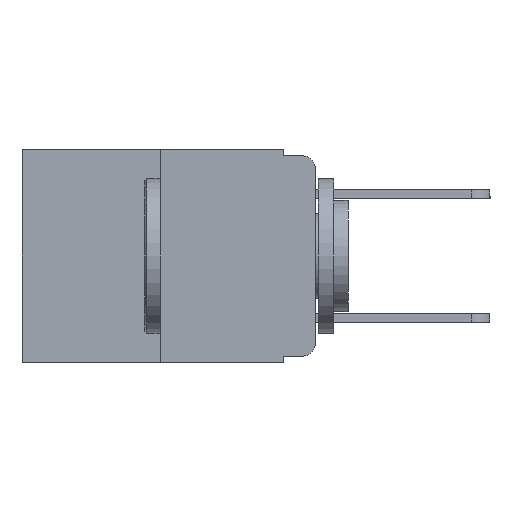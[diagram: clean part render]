
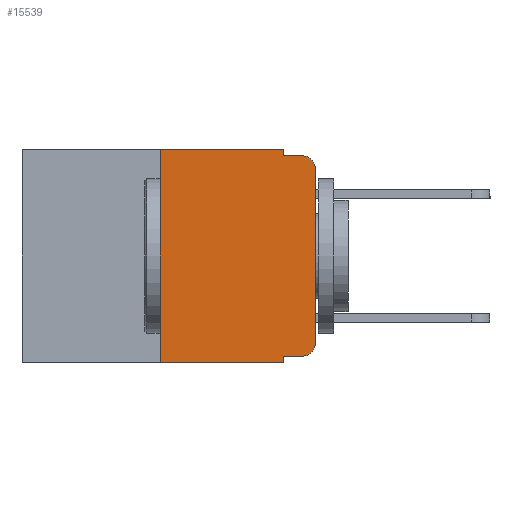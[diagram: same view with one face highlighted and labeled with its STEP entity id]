
A CAD part, left-side view. The second image highlights one B-rep face of the part: STEP entity #15539.
In plain terms, the highlighted planar face has unit normal (-1, 0, 0).
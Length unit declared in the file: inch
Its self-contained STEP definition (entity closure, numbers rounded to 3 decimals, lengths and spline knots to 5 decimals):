
#619 = CARTESIAN_POINT ( 'NONE',  ( 0., 0.02, -0.01 ) ) ;
#672 = VERTEX_POINT ( 'NONE', #3998 ) ;
#719 = VERTEX_POINT ( 'NONE', #619 ) ;
#890 = ORIENTED_EDGE ( 'NONE', *, *, #9875, .T. ) ;
#940 = CARTESIAN_POINT ( 'NONE',  ( 0., 0.051, -0.01 ) ) ;
#1463 = DIRECTION ( 'NONE',  ( -1., 0., 0. ) ) ;
#1755 = DIRECTION ( 'NONE',  ( 0., 0., -1. ) ) ;
#1847 = DIRECTION ( 'NONE',  ( -1., 0., 0. ) ) ;
#2084 = CARTESIAN_POINT ( 'NONE',  ( 0., 0.02, -0.03 ) ) ;
#2374 = LINE ( 'NONE', #5950, #15379 ) ;
#2557 = LINE ( 'NONE', #4442, #19301 ) ;
#2604 = CARTESIAN_POINT ( 'NONE',  ( 0., 0.25, -0.343 ) ) ;
#3172 = AXIS2_PLACEMENT_3D ( 'NONE', #11943, #1463, #13511 ) ;
#3240 = EDGE_CURVE ( 'NONE', #21312, #719, #14729, .T. ) ;
#3321 = PLANE ( 'NONE',  #15184 ) ;
#3429 = VECTOR ( 'NONE', #4644, 39.37008 ) ;
#3998 = CARTESIAN_POINT ( 'NONE',  ( 0., 0.02, -0.333 ) ) ;
#4213 = CARTESIAN_POINT ( 'NONE',  ( 0., 0.25, 0. ) ) ;
#4442 = CARTESIAN_POINT ( 'NONE',  ( 0., 0.051, 0. ) ) ;
#4644 = DIRECTION ( 'NONE',  ( 0., 0., -1. ) ) ;
#4833 = VERTEX_POINT ( 'NONE', #12881 ) ;
#5099 = DIRECTION ( 'NONE',  ( 1., 0., 0. ) ) ;
#5165 = VERTEX_POINT ( 'NONE', #5375 ) ;
#5375 = CARTESIAN_POINT ( 'NONE',  ( 0., 0.051, 0. ) ) ;
#5431 = ORIENTED_EDGE ( 'NONE', *, *, #12209, .T. ) ;
#5826 = ORIENTED_EDGE ( 'NONE', *, *, #19727, .T. ) ;
#5950 = CARTESIAN_POINT ( 'NONE',  ( 0., 0.25, 0. ) ) ;
#5953 = CARTESIAN_POINT ( 'NONE',  ( 0., 0.473, -0.343 ) ) ;
#5994 = CARTESIAN_POINT ( 'NONE',  ( 0., 0.051, -0.333 ) ) ;
#6104 = AXIS2_PLACEMENT_3D ( 'NONE', #2084, #1847, #1755 ) ;
#6261 = ORIENTED_EDGE ( 'NONE', *, *, #11265, .F. ) ;
#6351 = ORIENTED_EDGE ( 'NONE', *, *, #13387, .F. ) ;
#6363 = VERTEX_POINT ( 'NONE', #4213 ) ;
#6409 = ORIENTED_EDGE ( 'NONE', *, *, #3240, .T. ) ;
#6993 = CARTESIAN_POINT ( 'NONE',  ( 0., 0.051, -0.343 ) ) ;
#7061 = FACE_OUTER_BOUND ( 'NONE', #12437, .T. ) ;
#7512 = LINE ( 'NONE', #14798, #3429 ) ;
#7659 = CARTESIAN_POINT ( 'NONE',  ( 0., 0.473, 0. ) ) ;
#7741 = DIRECTION ( 'NONE',  ( 0., 0., 1. ) ) ;
#9471 = DIRECTION ( 'NONE',  ( 0., -1., 0. ) ) ;
#9743 = EDGE_CURVE ( 'NONE', #4833, #18101, #7512, .T. ) ;
#9875 = EDGE_CURVE ( 'NONE', #18501, #21312, #12802, .T. ) ;
#10159 = CARTESIAN_POINT ( 'NONE',  ( 0., 0., -0.313 ) ) ;
#10371 = DIRECTION ( 'NONE',  ( 0., 0., 1. ) ) ;
#10495 = CIRCLE ( 'NONE', #3172, 0.02 ) ;
#10674 = CARTESIAN_POINT ( 'NONE',  ( 0., 0.051, -0.01 ) ) ;
#11265 = EDGE_CURVE ( 'NONE', #5165, #17595, #2557, .T. ) ;
#11751 = LINE ( 'NONE', #940, #19759 ) ;
#11943 = CARTESIAN_POINT ( 'NONE',  ( 0., 0.02, -0.313 ) ) ;
#12209 = EDGE_CURVE ( 'NONE', #672, #18501, #10495, .T. ) ;
#12437 = EDGE_LOOP ( 'NONE', ( #890, #6409, #6351, #6261, #15819, #14343, #15837, #19990, #5826, #5431 ) ) ;
#12802 = LINE ( 'NONE', #21514, #17656 ) ;
#12881 = CARTESIAN_POINT ( 'NONE',  ( 0., 0.051, -0.333 ) ) ;
#13387 = EDGE_CURVE ( 'NONE', #17595, #719, #11751, .T. ) ;
#13511 = DIRECTION ( 'NONE',  ( 0., 0., -1. ) ) ;
#13616 = CARTESIAN_POINT ( 'NONE',  ( 0., 0.473, 0. ) ) ;
#14073 = CARTESIAN_POINT ( 'NONE',  ( 0., 0., -0.03 ) ) ;
#14343 = ORIENTED_EDGE ( 'NONE', *, *, #17214, .F. ) ;
#14729 = CIRCLE ( 'NONE', #6104, 0.02 ) ;
#14737 = DIRECTION ( 'NONE',  ( 0., -1., 0. ) ) ;
#14798 = CARTESIAN_POINT ( 'NONE',  ( 0., 0.051, 0. ) ) ;
#15184 = AXIS2_PLACEMENT_3D ( 'NONE', #13616, #5099, #16923 ) ;
#15379 = VECTOR ( 'NONE', #7741, 39.37008 ) ;
#15539 = ADVANCED_FACE ( 'NONE', ( #7061 ), #3321, .F. ) ;
#15819 = ORIENTED_EDGE ( 'NONE', *, *, #17189, .F. ) ;
#15837 = ORIENTED_EDGE ( 'NONE', *, *, #18880, .T. ) ;
#16193 = VECTOR ( 'NONE', #20798, 39.37008 ) ;
#16714 = LINE ( 'NONE', #5953, #16193 ) ;
#16923 = DIRECTION ( 'NONE',  ( 0., 0., -1. ) ) ;
#16930 = LINE ( 'NONE', #7659, #20121 ) ;
#17189 = EDGE_CURVE ( 'NONE', #6363, #5165, #16930, .T. ) ;
#17214 = EDGE_CURVE ( 'NONE', #18329, #6363, #2374, .T. ) ;
#17595 = VERTEX_POINT ( 'NONE', #10674 ) ;
#17656 = VECTOR ( 'NONE', #10371, 39.37008 ) ;
#18101 = VERTEX_POINT ( 'NONE', #6993 ) ;
#18162 = LINE ( 'NONE', #5994, #21299 ) ;
#18329 = VERTEX_POINT ( 'NONE', #2604 ) ;
#18501 = VERTEX_POINT ( 'NONE', #10159 ) ;
#18880 = EDGE_CURVE ( 'NONE', #18329, #18101, #16714, .T. ) ;
#19282 = DIRECTION ( 'NONE',  ( 0., -1., 0. ) ) ;
#19301 = VECTOR ( 'NONE', #19458, 39.37008 ) ;
#19458 = DIRECTION ( 'NONE',  ( 0., 0., -1. ) ) ;
#19727 = EDGE_CURVE ( 'NONE', #4833, #672, #18162, .T. ) ;
#19759 = VECTOR ( 'NONE', #14737, 39.37008 ) ;
#19990 = ORIENTED_EDGE ( 'NONE', *, *, #9743, .F. ) ;
#20121 = VECTOR ( 'NONE', #9471, 39.37008 ) ;
#20798 = DIRECTION ( 'NONE',  ( 0., -1., 0. ) ) ;
#21299 = VECTOR ( 'NONE', #19282, 39.37008 ) ;
#21312 = VERTEX_POINT ( 'NONE', #14073 ) ;
#21514 = CARTESIAN_POINT ( 'NONE',  ( 0., 0., 0. ) ) ;
